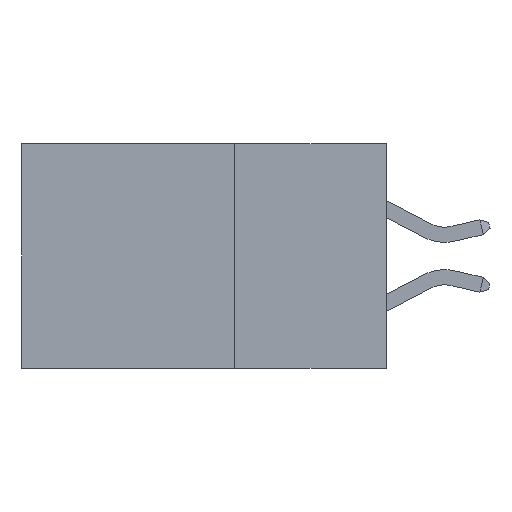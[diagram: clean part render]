
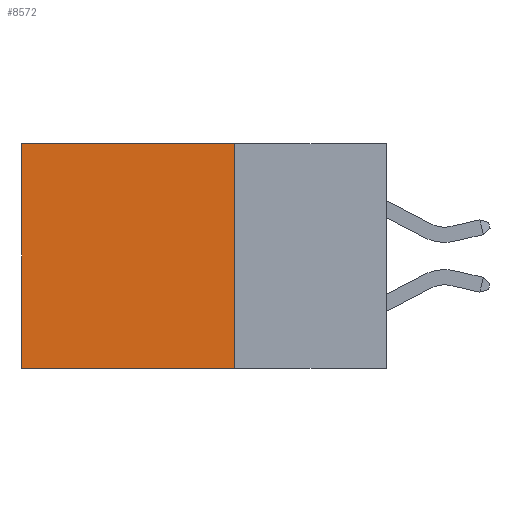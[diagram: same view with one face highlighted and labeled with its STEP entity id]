
A CAD part, left-side view. The second image highlights one B-rep face of the part: STEP entity #8572.
In plain terms, the highlighted planar face has unit normal (-1, 0, 0).
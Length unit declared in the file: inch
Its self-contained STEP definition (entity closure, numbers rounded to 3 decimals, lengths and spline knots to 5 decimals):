
#57 = VERTEX_POINT ( 'NONE', #3051 ) ;
#340 = LINE ( 'NONE', #6946, #9567 ) ;
#567 = CARTESIAN_POINT ( 'NONE',  ( 0.298, 0.25, 0. ) ) ;
#645 = AXIS2_PLACEMENT_3D ( 'NONE', #567, #1488, #7793 ) ;
#949 = CARTESIAN_POINT ( 'NONE',  ( 0.298, 0.6, -0.37 ) ) ;
#1265 = EDGE_CURVE ( 'NONE', #57, #10684, #1304, .T. ) ;
#1304 = LINE ( 'NONE', #3638, #8729 ) ;
#1488 = DIRECTION ( 'NONE',  ( 1., 0., 0. ) ) ;
#2745 = VERTEX_POINT ( 'NONE', #10185 ) ;
#3051 = CARTESIAN_POINT ( 'NONE',  ( 0.298, 0.25, 0. ) ) ;
#3305 = LINE ( 'NONE', #8454, #9943 ) ;
#3440 = EDGE_CURVE ( 'NONE', #2745, #4491, #3618, .T. ) ;
#3553 = DIRECTION ( 'NONE',  ( 0., 0., -1. ) ) ;
#3618 = LINE ( 'NONE', #6960, #5670 ) ;
#3638 = CARTESIAN_POINT ( 'NONE',  ( 0.298, 0.25, 0. ) ) ;
#3882 = CARTESIAN_POINT ( 'NONE',  ( 0.298, 0.25, -0.37 ) ) ;
#3893 = DIRECTION ( 'NONE',  ( 0., 0., -1. ) ) ;
#3935 = EDGE_CURVE ( 'NONE', #57, #2745, #3305, .T. ) ;
#4240 = ORIENTED_EDGE ( 'NONE', *, *, #8644, .F. ) ;
#4401 = ORIENTED_EDGE ( 'NONE', *, *, #3935, .T. ) ;
#4491 = VERTEX_POINT ( 'NONE', #949 ) ;
#5256 = DIRECTION ( 'NONE',  ( 0., 1., 0. ) ) ;
#5670 = VECTOR ( 'NONE', #3893, 39.37008 ) ;
#6072 = EDGE_LOOP ( 'NONE', ( #10706, #4240, #8566, #4401 ) ) ;
#6238 = DIRECTION ( 'NONE',  ( 0., 1., 0. ) ) ;
#6305 = FACE_OUTER_BOUND ( 'NONE', #6072, .T. ) ;
#6880 = PLANE ( 'NONE',  #645 ) ;
#6946 = CARTESIAN_POINT ( 'NONE',  ( 0.298, 0.25, -0.37 ) ) ;
#6960 = CARTESIAN_POINT ( 'NONE',  ( 0.298, 0.6, 0. ) ) ;
#7793 = DIRECTION ( 'NONE',  ( 0., 0., -1. ) ) ;
#8454 = CARTESIAN_POINT ( 'NONE',  ( 0.298, 0.25, 0. ) ) ;
#8566 = ORIENTED_EDGE ( 'NONE', *, *, #1265, .F. ) ;
#8572 = ADVANCED_FACE ( 'NONE', ( #6305 ), #6880, .F. ) ;
#8644 = EDGE_CURVE ( 'NONE', #10684, #4491, #340, .T. ) ;
#8729 = VECTOR ( 'NONE', #3553, 39.37008 ) ;
#9567 = VECTOR ( 'NONE', #5256, 39.37008 ) ;
#9943 = VECTOR ( 'NONE', #6238, 39.37008 ) ;
#10185 = CARTESIAN_POINT ( 'NONE',  ( 0.298, 0.6, 0. ) ) ;
#10684 = VERTEX_POINT ( 'NONE', #3882 ) ;
#10706 = ORIENTED_EDGE ( 'NONE', *, *, #3440, .T. ) ;
